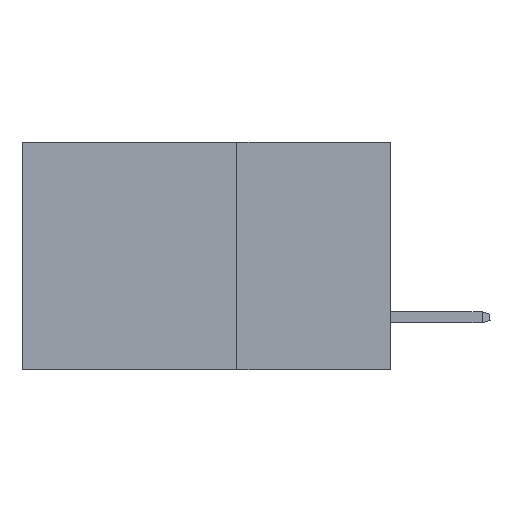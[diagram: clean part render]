
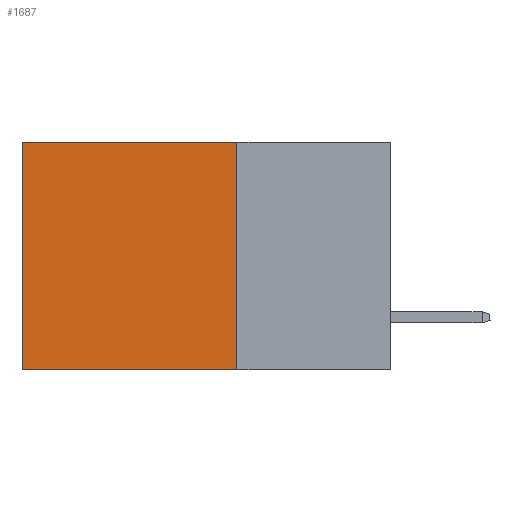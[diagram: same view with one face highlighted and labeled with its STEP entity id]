
A CAD part, left-side view. The second image highlights one B-rep face of the part: STEP entity #1687.
In plain terms, the highlighted planar face has unit normal (-1, 0, 0).
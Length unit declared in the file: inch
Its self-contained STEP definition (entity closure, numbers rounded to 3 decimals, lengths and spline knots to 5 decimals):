
#883 = DIRECTION ( 'NONE',  ( 0., 0., -1. ) ) ;
#1019 = LINE ( 'NONE', #9128, #6838 ) ;
#1687 = ADVANCED_FACE ( 'NONE', ( #19851 ), #6935, .F. ) ;
#1902 = EDGE_LOOP ( 'NONE', ( #22756, #22625, #4711, #19565 ) ) ;
#4711 = ORIENTED_EDGE ( 'NONE', *, *, #22621, .F. ) ;
#5014 = DIRECTION ( 'NONE',  ( 0., 1., 0. ) ) ;
#5020 = CARTESIAN_POINT ( 'NONE',  ( 0.2875, 0.6, -0.37 ) ) ;
#5678 = CARTESIAN_POINT ( 'NONE',  ( 0.2875, 0.25, -0.37 ) ) ;
#5996 = LINE ( 'NONE', #18287, #17699 ) ;
#6838 = VECTOR ( 'NONE', #5014, 39.37008 ) ;
#6935 = PLANE ( 'NONE',  #11747 ) ;
#8100 = LINE ( 'NONE', #14811, #22606 ) ;
#8888 = CARTESIAN_POINT ( 'NONE',  ( 0.2875, 0.6, 0. ) ) ;
#9128 = CARTESIAN_POINT ( 'NONE',  ( 0.2875, 0.25, -0.37 ) ) ;
#9180 = DIRECTION ( 'NONE',  ( 1., 0., 0. ) ) ;
#9933 = VECTOR ( 'NONE', #24373, 39.37008 ) ;
#10759 = DIRECTION ( 'NONE',  ( 0., 1., 0. ) ) ;
#11747 = AXIS2_PLACEMENT_3D ( 'NONE', #19057, #9180, #19141 ) ;
#13733 = VERTEX_POINT ( 'NONE', #5020 ) ;
#14234 = EDGE_CURVE ( 'NONE', #20636, #22104, #8100, .T. ) ;
#14811 = CARTESIAN_POINT ( 'NONE',  ( 0.2875, 0.25, 0. ) ) ;
#15169 = LINE ( 'NONE', #22314, #9933 ) ;
#17000 = EDGE_CURVE ( 'NONE', #23492, #13733, #1019, .T. ) ;
#17699 = VECTOR ( 'NONE', #883, 39.37008 ) ;
#18287 = CARTESIAN_POINT ( 'NONE',  ( 0.2875, 0.6, 0. ) ) ;
#19057 = CARTESIAN_POINT ( 'NONE',  ( 0.2875, 0.25, 0. ) ) ;
#19141 = DIRECTION ( 'NONE',  ( 0., 0., -1. ) ) ;
#19565 = ORIENTED_EDGE ( 'NONE', *, *, #14234, .T. ) ;
#19851 = FACE_OUTER_BOUND ( 'NONE', #1902, .T. ) ;
#20636 = VERTEX_POINT ( 'NONE', #21515 ) ;
#21515 = CARTESIAN_POINT ( 'NONE',  ( 0.2875, 0.25, 0. ) ) ;
#21549 = EDGE_CURVE ( 'NONE', #22104, #13733, #5996, .T. ) ;
#22104 = VERTEX_POINT ( 'NONE', #8888 ) ;
#22314 = CARTESIAN_POINT ( 'NONE',  ( 0.2875, 0.25, 0. ) ) ;
#22606 = VECTOR ( 'NONE', #10759, 39.37008 ) ;
#22621 = EDGE_CURVE ( 'NONE', #20636, #23492, #15169, .T. ) ;
#22625 = ORIENTED_EDGE ( 'NONE', *, *, #17000, .F. ) ;
#22756 = ORIENTED_EDGE ( 'NONE', *, *, #21549, .T. ) ;
#23492 = VERTEX_POINT ( 'NONE', #5678 ) ;
#24373 = DIRECTION ( 'NONE',  ( 0., 0., -1. ) ) ;
